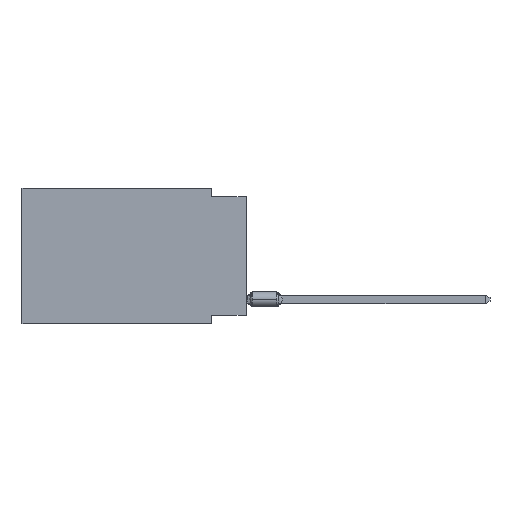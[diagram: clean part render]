
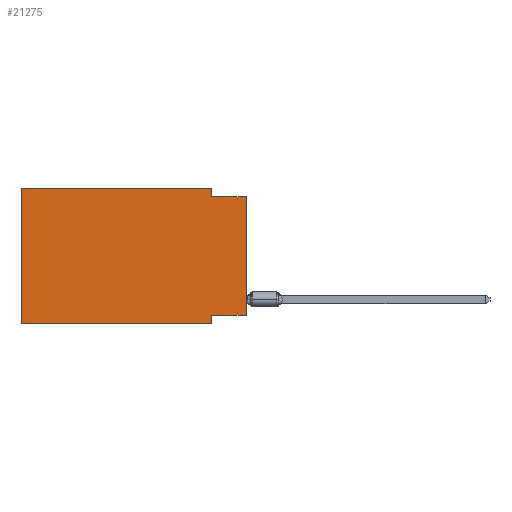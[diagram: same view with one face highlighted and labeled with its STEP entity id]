
A CAD part, left-side view. The second image highlights one B-rep face of the part: STEP entity #21275.
In plain terms, the highlighted planar face has unit normal (-1, 0, 0).
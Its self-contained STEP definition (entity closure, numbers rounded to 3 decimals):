
#176 = EDGE_CURVE ( 'NONE', #3836, #10198, #7810, .T. ) ;
#190 = DIRECTION ( 'NONE',  ( 0., 0., -1. ) ) ;
#248 = CARTESIAN_POINT ( 'NONE',  ( 0., 16.383, -9.906 ) ) ;
#1178 = LINE ( 'NONE', #15731, #21366 ) ;
#1666 = VECTOR ( 'NONE', #8545, 1000. ) ;
#1672 = VERTEX_POINT ( 'NONE', #8259 ) ;
#2085 = VECTOR ( 'NONE', #7262, 1000. ) ;
#2195 = DIRECTION ( 'NONE',  ( 0., 0., 1. ) ) ;
#2722 = CARTESIAN_POINT ( 'NONE',  ( 0., 2.54, 0. ) ) ;
#3488 = AXIS2_PLACEMENT_3D ( 'NONE', #14424, #26106, #16152 ) ;
#3526 = LINE ( 'NONE', #23607, #2085 ) ;
#3833 = ORIENTED_EDGE ( 'NONE', *, *, #7050, .T. ) ;
#3836 = VERTEX_POINT ( 'NONE', #23993 ) ;
#3985 = DIRECTION ( 'NONE',  ( 0., -1., 0. ) ) ;
#4508 = EDGE_CURVE ( 'NONE', #3836, #25186, #1178, .T. ) ;
#5462 = CARTESIAN_POINT ( 'NONE',  ( 0., 16.383, 0. ) ) ;
#5978 = LINE ( 'NONE', #14145, #9002 ) ;
#6210 = ORIENTED_EDGE ( 'NONE', *, *, #26433, .F. ) ;
#6981 = CARTESIAN_POINT ( 'NONE',  ( 0., 2.54, -9.906 ) ) ;
#7050 = EDGE_CURVE ( 'NONE', #1672, #20567, #16428, .T. ) ;
#7073 = EDGE_CURVE ( 'NONE', #10198, #20567, #18689, .T. ) ;
#7262 = DIRECTION ( 'NONE',  ( 0., -1., 0. ) ) ;
#7810 = LINE ( 'NONE', #17950, #20240 ) ;
#8259 = CARTESIAN_POINT ( 'NONE',  ( 0., 16.383, -9.906 ) ) ;
#8545 = DIRECTION ( 'NONE',  ( 0., 0., -1. ) ) ;
#8751 = VERTEX_POINT ( 'NONE', #26362 ) ;
#9002 = VECTOR ( 'NONE', #3985, 1000. ) ;
#10198 = VERTEX_POINT ( 'NONE', #22358 ) ;
#11559 = CARTESIAN_POINT ( 'NONE',  ( 0., 0., -0.635 ) ) ;
#11607 = DIRECTION ( 'NONE',  ( 0., 0., 1. ) ) ;
#11931 = DIRECTION ( 'NONE',  ( 0., 1., 0. ) ) ;
#12556 = CARTESIAN_POINT ( 'NONE',  ( 0., 2.54, -9.906 ) ) ;
#13436 = VERTEX_POINT ( 'NONE', #24532 ) ;
#14043 = ORIENTED_EDGE ( 'NONE', *, *, #23474, .F. ) ;
#14145 = CARTESIAN_POINT ( 'NONE',  ( 0., 16.383, 0. ) ) ;
#14424 = CARTESIAN_POINT ( 'NONE',  ( 0., 16.383, 0. ) ) ;
#14695 = DIRECTION ( 'NONE',  ( 0., -1., 0. ) ) ;
#14748 = LINE ( 'NONE', #2722, #20570 ) ;
#14763 = EDGE_CURVE ( 'NONE', #8751, #25186, #3526, .T. ) ;
#15448 = ORIENTED_EDGE ( 'NONE', *, *, #4508, .T. ) ;
#15731 = CARTESIAN_POINT ( 'NONE',  ( 0., 0., 0. ) ) ;
#16152 = DIRECTION ( 'NONE',  ( 0., 0., -1. ) ) ;
#16428 = LINE ( 'NONE', #248, #17888 ) ;
#17105 = VERTEX_POINT ( 'NONE', #5462 ) ;
#17888 = VECTOR ( 'NONE', #14695, 1000. ) ;
#17890 = PLANE ( 'NONE',  #3488 ) ;
#17950 = CARTESIAN_POINT ( 'NONE',  ( 0., 0., -9.271 ) ) ;
#18689 = LINE ( 'NONE', #12556, #1666 ) ;
#19056 = ORIENTED_EDGE ( 'NONE', *, *, #14763, .F. ) ;
#20240 = VECTOR ( 'NONE', #11931, 1000. ) ;
#20524 = CARTESIAN_POINT ( 'NONE',  ( 0., 16.383, 0. ) ) ;
#20567 = VERTEX_POINT ( 'NONE', #6981 ) ;
#20570 = VECTOR ( 'NONE', #190, 1000. ) ;
#21116 = VECTOR ( 'NONE', #2195, 1000. ) ;
#21275 = ADVANCED_FACE ( 'NONE', ( #23540 ), #17890, .F. ) ;
#21328 = ORIENTED_EDGE ( 'NONE', *, *, #176, .F. ) ;
#21366 = VECTOR ( 'NONE', #11607, 1000. ) ;
#22358 = CARTESIAN_POINT ( 'NONE',  ( 0., 2.54, -9.271 ) ) ;
#22564 = ORIENTED_EDGE ( 'NONE', *, *, #22942, .F. ) ;
#22942 = EDGE_CURVE ( 'NONE', #17105, #13436, #5978, .T. ) ;
#23474 = EDGE_CURVE ( 'NONE', #13436, #8751, #14748, .T. ) ;
#23540 = FACE_OUTER_BOUND ( 'NONE', #24911, .T. ) ;
#23607 = CARTESIAN_POINT ( 'NONE',  ( 0., 0., -0.635 ) ) ;
#23993 = CARTESIAN_POINT ( 'NONE',  ( 0., 0., -9.271 ) ) ;
#24532 = CARTESIAN_POINT ( 'NONE',  ( 0., 2.54, 0. ) ) ;
#24555 = LINE ( 'NONE', #20524, #21116 ) ;
#24911 = EDGE_LOOP ( 'NONE', ( #15448, #19056, #14043, #22564, #6210, #3833, #25641, #21328 ) ) ;
#25186 = VERTEX_POINT ( 'NONE', #11559 ) ;
#25641 = ORIENTED_EDGE ( 'NONE', *, *, #7073, .F. ) ;
#26106 = DIRECTION ( 'NONE',  ( 1., 0., 0. ) ) ;
#26362 = CARTESIAN_POINT ( 'NONE',  ( 0., 2.54, -0.635 ) ) ;
#26433 = EDGE_CURVE ( 'NONE', #1672, #17105, #24555, .T. ) ;
